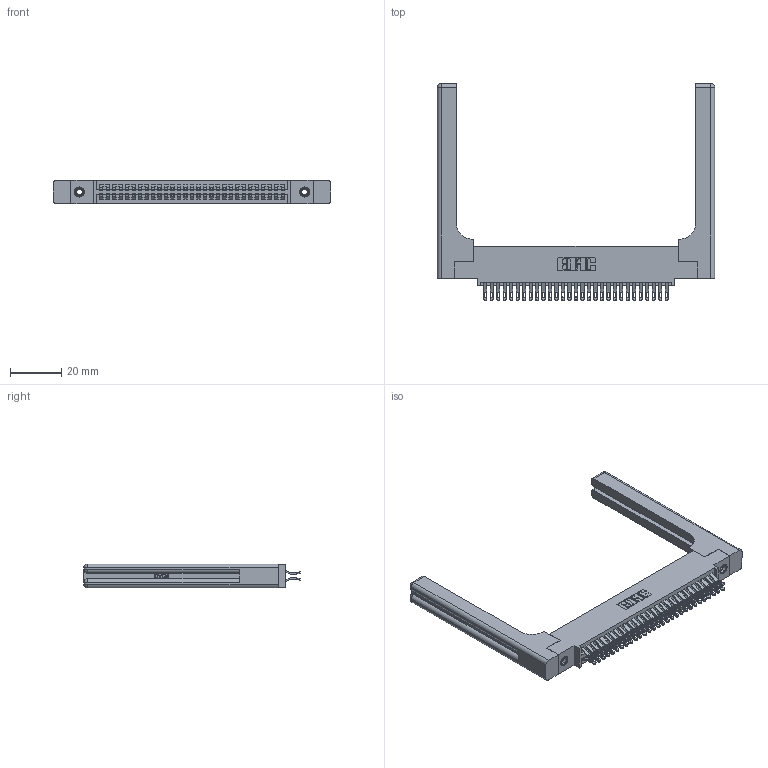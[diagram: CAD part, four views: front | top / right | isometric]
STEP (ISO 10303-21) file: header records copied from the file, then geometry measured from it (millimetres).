
FILE_DESCRIPTION (( 'STEP AP203' ), '1' );
FILE_NAME ('395-058-555-558.STEP', '2019-10-23T12:44:09', ( '' ), ( '' ), 'SwSTEP 2.0', 'SolidWorks 2016', '' );
FILE_SCHEMA (( 'CONFIG_CONTROL_DESIGN' ));
Length unit declared in the file: inch
Products named in the file (5): 345-220-058_345-220-058; 395-058-555-558; 345 Part_0.110 Offset - 0.156 Dia-TH; 345-292-001_555 Tail; 345-250-001_345-250-001-102
Assembly tree (63 placements, depth 2):
  395-058-555-558
    345 Part_0.110 Offset - 0.156 Dia-TH
    345-292-001_555 Tail  x58
    345-250-001_345-250-001-102  x2
    345-220-058_345-220-058  x2
Bounding box: 108.69 x 84.89 x 9.4 mm (x, y, z)
Volume: 19007.2 mm3; surface area: 21053.3 mm2
Topology: 63 solids, 63 shells, 3634 faces, 11285 edges, 7502 vertices
Faces by surface type: plane 2030, cylinder 1544, bspline 36, cone 12, sphere 8, torus 4
Entity records: 30144 total; most frequent: CARTESIAN_POINT 6095, ORIENTED_EDGE 4796, DIRECTION 4290, EDGE_CURVE 2398, VECTOR 2038, LINE 2038, VERTEX_POINT 1590, AXIS2_PLACEMENT_3D 1126
